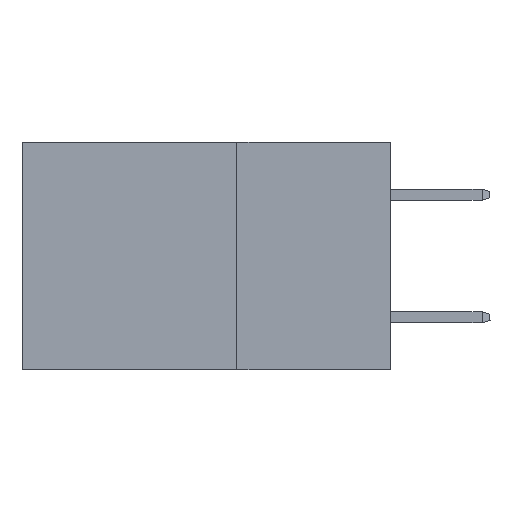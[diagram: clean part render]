
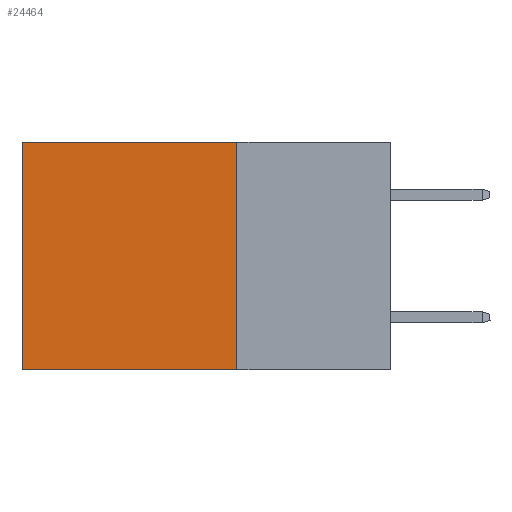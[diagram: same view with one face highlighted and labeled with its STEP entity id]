
A CAD part, left-side view. The second image highlights one B-rep face of the part: STEP entity #24464.
In plain terms, the highlighted planar face has unit normal (-1, 0, 0).
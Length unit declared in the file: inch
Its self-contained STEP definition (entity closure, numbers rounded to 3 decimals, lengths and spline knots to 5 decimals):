
#1818 = VECTOR ( 'NONE', #3761, 39.37008 ) ;
#3034 = DIRECTION ( 'NONE',  ( 0., 1., 0. ) ) ;
#3239 = CARTESIAN_POINT ( 'NONE',  ( 0.2875, 0.25, -0.37 ) ) ;
#3485 = CARTESIAN_POINT ( 'NONE',  ( 0.2875, 0.25, -0.37 ) ) ;
#3761 = DIRECTION ( 'NONE',  ( 0., 0., -1. ) ) ;
#3986 = VECTOR ( 'NONE', #9184, 39.37008 ) ;
#5052 = CARTESIAN_POINT ( 'NONE',  ( 0.2875, 0.6, -0.37 ) ) ;
#5250 = VECTOR ( 'NONE', #24117, 39.37008 ) ;
#5386 = PLANE ( 'NONE',  #9742 ) ;
#5562 = VERTEX_POINT ( 'NONE', #23352 ) ;
#5884 = ORIENTED_EDGE ( 'NONE', *, *, #24500, .F. ) ;
#7054 = LINE ( 'NONE', #24056, #1818 ) ;
#8528 = ORIENTED_EDGE ( 'NONE', *, *, #9155, .F. ) ;
#9155 = EDGE_CURVE ( 'NONE', #26896, #9349, #21944, .T. ) ;
#9184 = DIRECTION ( 'NONE',  ( 0., 0., -1. ) ) ;
#9349 = VERTEX_POINT ( 'NONE', #3485 ) ;
#9742 = AXIS2_PLACEMENT_3D ( 'NONE', #11859, #23426, #12153 ) ;
#10306 = CARTESIAN_POINT ( 'NONE',  ( 0.2875, 0.25, 0. ) ) ;
#10514 = ORIENTED_EDGE ( 'NONE', *, *, #21191, .T. ) ;
#11859 = CARTESIAN_POINT ( 'NONE',  ( 0.2875, 0.25, 0. ) ) ;
#12153 = DIRECTION ( 'NONE',  ( 0., 0., -1. ) ) ;
#12966 = LINE ( 'NONE', #10306, #5250 ) ;
#13777 = CARTESIAN_POINT ( 'NONE',  ( 0.2875, 0.25, 0. ) ) ;
#14019 = ORIENTED_EDGE ( 'NONE', *, *, #20053, .T. ) ;
#14837 = VECTOR ( 'NONE', #3034, 39.37008 ) ;
#17269 = LINE ( 'NONE', #3239, #14837 ) ;
#19734 = FACE_OUTER_BOUND ( 'NONE', #24896, .T. ) ;
#20053 = EDGE_CURVE ( 'NONE', #5562, #27247, #7054, .T. ) ;
#21191 = EDGE_CURVE ( 'NONE', #26896, #5562, #12966, .T. ) ;
#21944 = LINE ( 'NONE', #13777, #3986 ) ;
#23352 = CARTESIAN_POINT ( 'NONE',  ( 0.2875, 0.6, 0. ) ) ;
#23426 = DIRECTION ( 'NONE',  ( 1., 0., 0. ) ) ;
#24056 = CARTESIAN_POINT ( 'NONE',  ( 0.2875, 0.6, 0. ) ) ;
#24117 = DIRECTION ( 'NONE',  ( 0., 1., 0. ) ) ;
#24464 = ADVANCED_FACE ( 'NONE', ( #19734 ), #5386, .F. ) ;
#24500 = EDGE_CURVE ( 'NONE', #9349, #27247, #17269, .T. ) ;
#24774 = CARTESIAN_POINT ( 'NONE',  ( 0.2875, 0.25, 0. ) ) ;
#24896 = EDGE_LOOP ( 'NONE', ( #14019, #5884, #8528, #10514 ) ) ;
#26896 = VERTEX_POINT ( 'NONE', #24774 ) ;
#27247 = VERTEX_POINT ( 'NONE', #5052 ) ;
